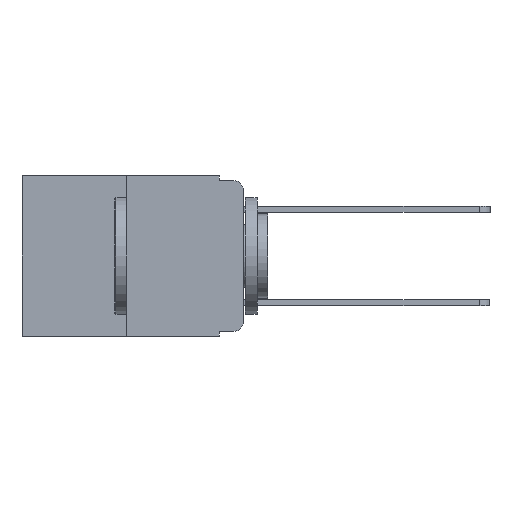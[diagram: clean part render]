
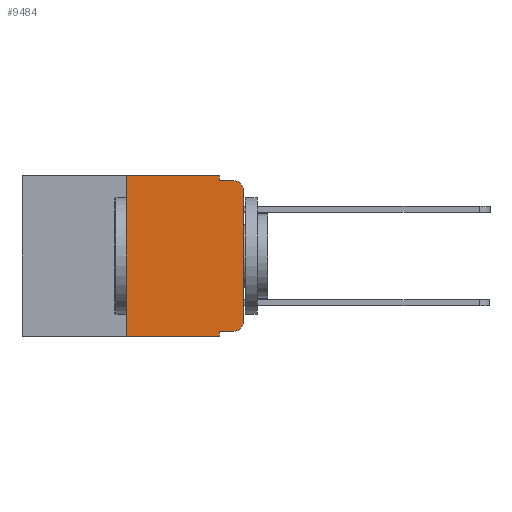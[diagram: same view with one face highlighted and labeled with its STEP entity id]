
A CAD part, left-side view. The second image highlights one B-rep face of the part: STEP entity #9484.
In plain terms, the highlighted planar face has unit normal (-1, 0, 0).
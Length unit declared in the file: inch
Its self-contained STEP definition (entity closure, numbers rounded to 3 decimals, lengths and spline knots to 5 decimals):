
#278 = DIRECTION ( 'NONE',  ( 0., 0., -1. ) ) ;
#328 = CARTESIAN_POINT ( 'NONE',  ( 0., 0.051, 0. ) ) ;
#461 = ORIENTED_EDGE ( 'NONE', *, *, #14095, .T. ) ;
#877 = ORIENTED_EDGE ( 'NONE', *, *, #4188, .T. ) ;
#1154 = VERTEX_POINT ( 'NONE', #2608 ) ;
#1287 = ORIENTED_EDGE ( 'NONE', *, *, #5146, .T. ) ;
#1371 = VERTEX_POINT ( 'NONE', #13713 ) ;
#1423 = LINE ( 'NONE', #13086, #12188 ) ;
#1476 = LINE ( 'NONE', #12680, #9547 ) ;
#1646 = ORIENTED_EDGE ( 'NONE', *, *, #12568, .T. ) ;
#1767 = CIRCLE ( 'NONE', #16803, 0.02 ) ;
#1802 = VERTEX_POINT ( 'NONE', #13091 ) ;
#2300 = DIRECTION ( 'NONE',  ( 0., -1., 0. ) ) ;
#2306 = ORIENTED_EDGE ( 'NONE', *, *, #14541, .F. ) ;
#2584 = DIRECTION ( 'NONE',  ( 1., 0., 0. ) ) ;
#2608 = CARTESIAN_POINT ( 'NONE',  ( 0., 0., -0.03 ) ) ;
#2648 = VERTEX_POINT ( 'NONE', #13410 ) ;
#3305 = ORIENTED_EDGE ( 'NONE', *, *, #12352, .T. ) ;
#3620 = VERTEX_POINT ( 'NONE', #16372 ) ;
#3946 = ORIENTED_EDGE ( 'NONE', *, *, #9688, .F. ) ;
#4188 = EDGE_CURVE ( 'NONE', #8349, #1371, #12741, .T. ) ;
#4721 = EDGE_LOOP ( 'NONE', ( #461, #3305, #5547, #3946, #2306, #7491, #1646, #6703, #1287, #877 ) ) ;
#4760 = DIRECTION ( 'NONE',  ( 0., -1., 0. ) ) ;
#4979 = VERTEX_POINT ( 'NONE', #14445 ) ;
#4994 = VERTEX_POINT ( 'NONE', #12504 ) ;
#5146 = EDGE_CURVE ( 'NONE', #1802, #8349, #6018, .T. ) ;
#5348 = AXIS2_PLACEMENT_3D ( 'NONE', #9706, #9768, #9650 ) ;
#5360 = DIRECTION ( 'NONE',  ( 0., 0., 1. ) ) ;
#5547 = ORIENTED_EDGE ( 'NONE', *, *, #11429, .F. ) ;
#5606 = VECTOR ( 'NONE', #7299, 39.37008 ) ;
#5676 = CARTESIAN_POINT ( 'NONE',  ( 0., 0.02, -0.333 ) ) ;
#5885 = AXIS2_PLACEMENT_3D ( 'NONE', #12146, #2584, #12208 ) ;
#6018 = LINE ( 'NONE', #11191, #6434 ) ;
#6434 = VECTOR ( 'NONE', #11171, 39.37008 ) ;
#6600 = CARTESIAN_POINT ( 'NONE',  ( 0., 0.051, -0.01 ) ) ;
#6703 = ORIENTED_EDGE ( 'NONE', *, *, #6956, .F. ) ;
#6783 = CARTESIAN_POINT ( 'NONE',  ( 0., 0.25, 0. ) ) ;
#6956 = EDGE_CURVE ( 'NONE', #1802, #4994, #12269, .T. ) ;
#7102 = CARTESIAN_POINT ( 'NONE',  ( 0., 0.02, -0.03 ) ) ;
#7299 = DIRECTION ( 'NONE',  ( 0., 0., -1. ) ) ;
#7371 = DIRECTION ( 'NONE',  ( 0., -1., 0. ) ) ;
#7491 = ORIENTED_EDGE ( 'NONE', *, *, #8790, .F. ) ;
#7794 = DIRECTION ( 'NONE',  ( 0., 0., 1. ) ) ;
#8349 = VERTEX_POINT ( 'NONE', #5676 ) ;
#8475 = DIRECTION ( 'NONE',  ( 0., 0., -1. ) ) ;
#8741 = VECTOR ( 'NONE', #278, 39.37008 ) ;
#8790 = EDGE_CURVE ( 'NONE', #3620, #4979, #11492, .T. ) ;
#9484 = ADVANCED_FACE ( 'NONE', ( #16418 ), #10849, .F. ) ;
#9547 = VECTOR ( 'NONE', #7371, 39.37008 ) ;
#9556 = LINE ( 'NONE', #16778, #16113 ) ;
#9650 = DIRECTION ( 'NONE',  ( 0., 0., -1. ) ) ;
#9688 = EDGE_CURVE ( 'NONE', #12876, #2648, #12731, .T. ) ;
#9706 = CARTESIAN_POINT ( 'NONE',  ( 0., 0.02, -0.313 ) ) ;
#9768 = DIRECTION ( 'NONE',  ( -1., 0., 0. ) ) ;
#10694 = CARTESIAN_POINT ( 'NONE',  ( 0., 0.051, 0. ) ) ;
#10701 = VERTEX_POINT ( 'NONE', #11640 ) ;
#10849 = PLANE ( 'NONE',  #5885 ) ;
#11171 = DIRECTION ( 'NONE',  ( 0., -1., 0. ) ) ;
#11191 = CARTESIAN_POINT ( 'NONE',  ( 0., 0.051, -0.333 ) ) ;
#11211 = VECTOR ( 'NONE', #2300, 39.37008 ) ;
#11244 = CARTESIAN_POINT ( 'NONE',  ( 0., 0.051, 0. ) ) ;
#11429 = EDGE_CURVE ( 'NONE', #2648, #10701, #11641, .T. ) ;
#11492 = LINE ( 'NONE', #6783, #15805 ) ;
#11640 = CARTESIAN_POINT ( 'NONE',  ( 0., 0.02, -0.01 ) ) ;
#11641 = LINE ( 'NONE', #6600, #11211 ) ;
#12146 = CARTESIAN_POINT ( 'NONE',  ( 0., 0.473, 0. ) ) ;
#12188 = VECTOR ( 'NONE', #7794, 39.37008 ) ;
#12208 = DIRECTION ( 'NONE',  ( 0., 0., -1. ) ) ;
#12269 = LINE ( 'NONE', #328, #8741 ) ;
#12352 = EDGE_CURVE ( 'NONE', #1154, #10701, #1767, .T. ) ;
#12504 = CARTESIAN_POINT ( 'NONE',  ( 0., 0.051, -0.343 ) ) ;
#12568 = EDGE_CURVE ( 'NONE', #3620, #4994, #9556, .T. ) ;
#12680 = CARTESIAN_POINT ( 'NONE',  ( 0., 0.473, 0. ) ) ;
#12731 = LINE ( 'NONE', #11244, #5606 ) ;
#12741 = CIRCLE ( 'NONE', #5348, 0.02 ) ;
#12876 = VERTEX_POINT ( 'NONE', #10694 ) ;
#13086 = CARTESIAN_POINT ( 'NONE',  ( 0., 0., 0. ) ) ;
#13091 = CARTESIAN_POINT ( 'NONE',  ( 0., 0.051, -0.333 ) ) ;
#13410 = CARTESIAN_POINT ( 'NONE',  ( 0., 0.051, -0.01 ) ) ;
#13713 = CARTESIAN_POINT ( 'NONE',  ( 0., 0., -0.313 ) ) ;
#14095 = EDGE_CURVE ( 'NONE', #1371, #1154, #1423, .T. ) ;
#14445 = CARTESIAN_POINT ( 'NONE',  ( 0., 0.25, 0. ) ) ;
#14541 = EDGE_CURVE ( 'NONE', #4979, #12876, #1476, .T. ) ;
#15805 = VECTOR ( 'NONE', #5360, 39.37008 ) ;
#16113 = VECTOR ( 'NONE', #4760, 39.37008 ) ;
#16365 = DIRECTION ( 'NONE',  ( -1., 0., 0. ) ) ;
#16372 = CARTESIAN_POINT ( 'NONE',  ( 0., 0.25, -0.343 ) ) ;
#16418 = FACE_OUTER_BOUND ( 'NONE', #4721, .T. ) ;
#16778 = CARTESIAN_POINT ( 'NONE',  ( 0., 0.473, -0.343 ) ) ;
#16803 = AXIS2_PLACEMENT_3D ( 'NONE', #7102, #16365, #8475 ) ;
